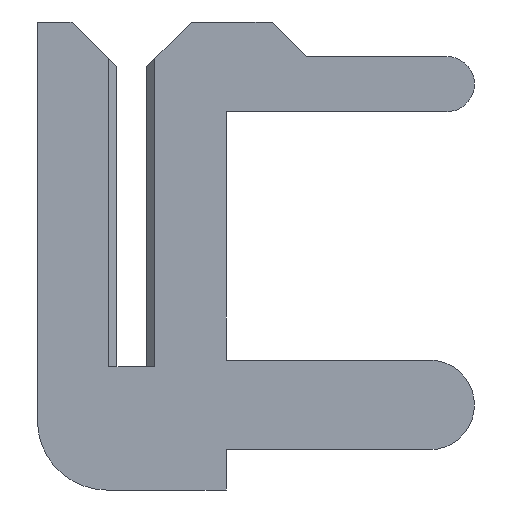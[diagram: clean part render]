
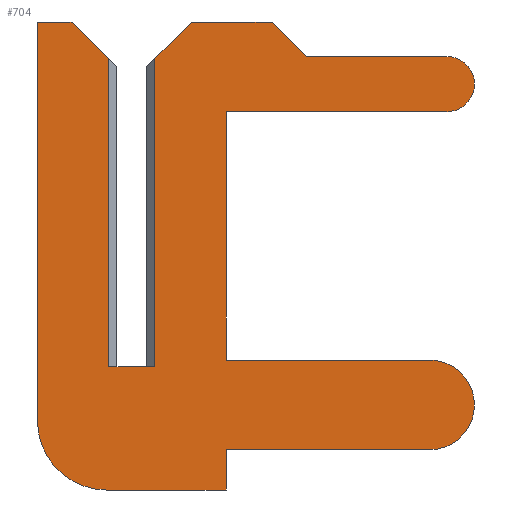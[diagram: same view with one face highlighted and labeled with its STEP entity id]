
A CAD part, left-side view. The second image highlights one B-rep face of the part: STEP entity #704.
In plain terms, the highlighted planar face has unit normal (-1, 0, 0).
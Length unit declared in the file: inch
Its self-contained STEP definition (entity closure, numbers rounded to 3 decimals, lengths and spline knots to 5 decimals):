
#10 = DIRECTION ( 'NONE',  ( 0., -1., 0. ) ) ;
#14 = ORIENTED_EDGE ( 'NONE', *, *, #874, .F. ) ;
#32 = PLANE ( 'NONE',  #618 ) ;
#52 = VERTEX_POINT ( 'NONE', #61 ) ;
#55 = EDGE_CURVE ( 'NONE', #274, #989, #487, .T. ) ;
#57 = VECTOR ( 'NONE', #414, 39.37008 ) ;
#61 = CARTESIAN_POINT ( 'NONE',  ( -0.01, -0.01, 0.134 ) ) ;
#77 = CARTESIAN_POINT ( 'NONE',  ( -0.01, -0.1295, 0.003 ) ) ;
#81 = VERTEX_POINT ( 'NONE', #761 ) ;
#87 = AXIS2_PLACEMENT_3D ( 'NONE', #1028, #701, #204 ) ;
#99 = DIRECTION ( 'NONE',  ( 0., 0., 1. ) ) ;
#117 = LINE ( 'NONE', #719, #149 ) ;
#140 = VECTOR ( 'NONE', #871, 39.37008 ) ;
#149 = VECTOR ( 'NONE', #219, 39.37008 ) ;
#153 = LINE ( 'NONE', #344, #800 ) ;
#162 = VERTEX_POINT ( 'NONE', #771 ) ;
#165 = DIRECTION ( 'NONE',  ( 0., 0., 1. ) ) ;
#181 = ORIENTED_EDGE ( 'NONE', *, *, #519, .F. ) ;
#186 = LINE ( 'NONE', #328, #364 ) ;
#188 = CARTESIAN_POINT ( 'NONE',  ( -0.01, -0.01, 0.15 ) ) ;
#191 = CARTESIAN_POINT ( 'NONE',  ( -0.01, -0.041, -0.0535 ) ) ;
#192 = CARTESIAN_POINT ( 'NONE',  ( -0.01, 0.01, 0. ) ) ;
#195 = VERTEX_POINT ( 'NONE', #383 ) ;
#197 = VERTEX_POINT ( 'NONE', #1095 ) ;
#199 = ORIENTED_EDGE ( 'NONE', *, *, #672, .F. ) ;
#200 = CIRCLE ( 'NONE', #1031, 0.012 ) ;
#204 = DIRECTION ( 'NONE',  ( 0., 0., 1. ) ) ;
#212 = CARTESIAN_POINT ( 'NONE',  ( -0.01, -0.041, -0.0535 ) ) ;
#213 = VECTOR ( 'NONE', #10, 39.37008 ) ;
#219 = DIRECTION ( 'NONE',  ( 0., 1., 0. ) ) ;
#226 = DIRECTION ( 'NONE',  ( 0., 1., 0. ) ) ;
#237 = DIRECTION ( 'NONE',  ( 0., 0., 1. ) ) ;
#272 = DIRECTION ( 'NONE',  ( 0., -0.707, -0.707 ) ) ;
#274 = VERTEX_POINT ( 'NONE', #192 ) ;
#275 = VERTEX_POINT ( 'NONE', #1210 ) ;
#299 = EDGE_CURVE ( 'NONE', #275, #1102, #401, .T. ) ;
#300 = CARTESIAN_POINT ( 'NONE',  ( -0.01, -0.137, 0.111 ) ) ;
#313 = VECTOR ( 'NONE', #165, 39.37008 ) ;
#328 = CARTESIAN_POINT ( 'NONE',  ( -0.01, -0.076, 0.135 ) ) ;
#343 = ORIENTED_EDGE ( 'NONE', *, *, #1260, .F. ) ;
#344 = CARTESIAN_POINT ( 'NONE',  ( -0.01, -0.041, -0.036 ) ) ;
#353 = LINE ( 'NONE', #1224, #926 ) ;
#364 = VECTOR ( 'NONE', #1034, 39.37008 ) ;
#368 = CARTESIAN_POINT ( 'NONE',  ( -0.01, 0.0065, 0.1305 ) ) ;
#369 = VECTOR ( 'NONE', #1001, 39.37008 ) ;
#370 = DIRECTION ( 'NONE',  ( 0., -1., 0. ) ) ;
#371 = ORIENTED_EDGE ( 'NONE', *, *, #504, .T. ) ;
#383 = CARTESIAN_POINT ( 'NONE',  ( -0.01, 0.041, -0.0235 ) ) ;
#384 = ORIENTED_EDGE ( 'NONE', *, *, #547, .F. ) ;
#391 = VECTOR ( 'NONE', #1147, 39.37008 ) ;
#394 = CARTESIAN_POINT ( 'NONE',  ( -0.01, -0.137, 0.123 ) ) ;
#401 = LINE ( 'NONE', #77, #369 ) ;
#414 = DIRECTION ( 'NONE',  ( 0., 0., -1. ) ) ;
#419 = ORIENTED_EDGE ( 'NONE', *, *, #739, .F. ) ;
#421 = DIRECTION ( 'NONE',  ( 0., 0., -1. ) ) ;
#441 = ORIENTED_EDGE ( 'NONE', *, *, #55, .F. ) ;
#444 = CARTESIAN_POINT ( 'NONE',  ( -0.01, 0.011, -0.0235 ) ) ;
#462 = LINE ( 'NONE', #1049, #391 ) ;
#477 = LINE ( 'NONE', #368, #671 ) ;
#487 = LINE ( 'NONE', #961, #140 ) ;
#496 = LINE ( 'NONE', #188, #864 ) ;
#504 = EDGE_CURVE ( 'NONE', #274, #162, #582, .T. ) ;
#518 = VERTEX_POINT ( 'NONE', #1127 ) ;
#519 = EDGE_CURVE ( 'NONE', #1248, #1035, #353, .T. ) ;
#530 = VERTEX_POINT ( 'NONE', #1228 ) ;
#547 = EDGE_CURVE ( 'NONE', #791, #1081, #568, .T. ) ;
#565 = EDGE_LOOP ( 'NONE', ( #1098, #603, #441, #371, #819, #181, #14, #636, #419, #384, #1231, #709, #652, #199, #638, #726, #343, #1037, #821 ) ) ;
#568 = LINE ( 'NONE', #212, #57 ) ;
#570 = CARTESIAN_POINT ( 'NONE',  ( -0.01, -0.1295, -0.036 ) ) ;
#582 = LINE ( 'NONE', #900, #1268 ) ;
#603 = ORIENTED_EDGE ( 'NONE', *, *, #1197, .T. ) ;
#605 = EDGE_CURVE ( 'NONE', #1102, #953, #891, .T. ) ;
#618 = AXIS2_PLACEMENT_3D ( 'NONE', #444, #660, #237 ) ;
#636 = ORIENTED_EDGE ( 'NONE', *, *, #1267, .F. ) ;
#638 = ORIENTED_EDGE ( 'NONE', *, *, #1160, .F. ) ;
#644 = LINE ( 'NONE', #1236, #213 ) ;
#652 = ORIENTED_EDGE ( 'NONE', *, *, #299, .F. ) ;
#660 = DIRECTION ( 'NONE',  ( -1., 0., 0. ) ) ;
#670 = VERTEX_POINT ( 'NONE', #905 ) ;
#671 = VECTOR ( 'NONE', #272, 39.37008 ) ;
#672 = EDGE_CURVE ( 'NONE', #530, #275, #994, .T. ) ;
#675 = VECTOR ( 'NONE', #883, 39.37008 ) ;
#701 = DIRECTION ( 'NONE',  ( 1., 0., 0. ) ) ;
#704 = ADVANCED_FACE ( 'NONE', ( #711 ), #32, .T. ) ;
#706 = EDGE_CURVE ( 'NONE', #52, #518, #462, .T. ) ;
#709 = ORIENTED_EDGE ( 'NONE', *, *, #605, .F. ) ;
#711 = FACE_OUTER_BOUND ( 'NONE', #565, .T. ) ;
#719 = CARTESIAN_POINT ( 'NONE',  ( -0.01, 0.011, -0.0535 ) ) ;
#726 = ORIENTED_EDGE ( 'NONE', *, *, #1062, .F. ) ;
#738 = CARTESIAN_POINT ( 'NONE',  ( -0.01, -0.041, 0.003 ) ) ;
#739 = EDGE_CURVE ( 'NONE', #1081, #744, #117, .T. ) ;
#744 = VERTEX_POINT ( 'NONE', #1040 ) ;
#761 = CARTESIAN_POINT ( 'NONE',  ( -0.01, -0.137, 0.135 ) ) ;
#764 = CARTESIAN_POINT ( 'NONE',  ( -0.01, -0.026, 0.15 ) ) ;
#767 = VECTOR ( 'NONE', #370, 39.37008 ) ;
#771 = CARTESIAN_POINT ( 'NONE',  ( -0.01, 0.01, 0.134 ) ) ;
#785 = CARTESIAN_POINT ( 'NONE',  ( -0.01, -0.041, 0.111 ) ) ;
#791 = VERTEX_POINT ( 'NONE', #940 ) ;
#798 = EDGE_CURVE ( 'NONE', #670, #197, #186, .T. ) ;
#800 = VECTOR ( 'NONE', #226, 39.37008 ) ;
#808 = DIRECTION ( 'NONE',  ( 0., 0., 1. ) ) ;
#819 = ORIENTED_EDGE ( 'NONE', *, *, #968, .F. ) ;
#821 = ORIENTED_EDGE ( 'NONE', *, *, #830, .F. ) ;
#826 = LINE ( 'NONE', #764, #767 ) ;
#830 = EDGE_CURVE ( 'NONE', #518, #670, #826, .T. ) ;
#864 = VECTOR ( 'NONE', #421, 39.37008 ) ;
#866 = CARTESIAN_POINT ( 'NONE',  ( -0.01, 0.041, 0.15 ) ) ;
#871 = DIRECTION ( 'NONE',  ( 0., -1., 0. ) ) ;
#874 = EDGE_CURVE ( 'NONE', #195, #1248, #1285, .T. ) ;
#883 = DIRECTION ( 'NONE',  ( 0., 1., 0. ) ) ;
#891 = CIRCLE ( 'NONE', #1150, 0.0195 ) ;
#898 = CARTESIAN_POINT ( 'NONE',  ( -0.01, -0.1295, 0.003 ) ) ;
#900 = CARTESIAN_POINT ( 'NONE',  ( -0.01, 0.01, -0.0235 ) ) ;
#905 = CARTESIAN_POINT ( 'NONE',  ( -0.01, -0.061, 0.15 ) ) ;
#910 = CARTESIAN_POINT ( 'NONE',  ( -0.01, 0.041, 0.15 ) ) ;
#926 = VECTOR ( 'NONE', #1220, 39.37008 ) ;
#940 = CARTESIAN_POINT ( 'NONE',  ( -0.01, -0.041, -0.036 ) ) ;
#953 = VERTEX_POINT ( 'NONE', #570 ) ;
#961 = CARTESIAN_POINT ( 'NONE',  ( -0.01, 0.0065, 0. ) ) ;
#968 = EDGE_CURVE ( 'NONE', #1035, #162, #477, .T. ) ;
#989 = VERTEX_POINT ( 'NONE', #1008 ) ;
#994 = LINE ( 'NONE', #738, #1011 ) ;
#1001 = DIRECTION ( 'NONE',  ( 0., -1., 0. ) ) ;
#1003 = DIRECTION ( 'NONE',  ( 0., 0., 1. ) ) ;
#1008 = CARTESIAN_POINT ( 'NONE',  ( -0.01, -0.01, 0. ) ) ;
#1011 = VECTOR ( 'NONE', #1237, 39.37008 ) ;
#1024 = CARTESIAN_POINT ( 'NONE',  ( -0.01, -0.1295, -0.0165 ) ) ;
#1028 = CARTESIAN_POINT ( 'NONE',  ( -0.01, 0.011, -0.0235 ) ) ;
#1031 = AXIS2_PLACEMENT_3D ( 'NONE', #394, #1100, #1003 ) ;
#1034 = DIRECTION ( 'NONE',  ( 0., -0.707, -0.707 ) ) ;
#1035 = VERTEX_POINT ( 'NONE', #1090 ) ;
#1037 = ORIENTED_EDGE ( 'NONE', *, *, #798, .F. ) ;
#1040 = CARTESIAN_POINT ( 'NONE',  ( -0.01, 0.011, -0.0535 ) ) ;
#1049 = CARTESIAN_POINT ( 'NONE',  ( -0.01, -0.0065, 0.1305 ) ) ;
#1062 = EDGE_CURVE ( 'NONE', #81, #1245, #200, .T. ) ;
#1081 = VERTEX_POINT ( 'NONE', #191 ) ;
#1090 = CARTESIAN_POINT ( 'NONE',  ( -0.01, 0.026, 0.15 ) ) ;
#1095 = CARTESIAN_POINT ( 'NONE',  ( -0.01, -0.076, 0.135 ) ) ;
#1098 = ORIENTED_EDGE ( 'NONE', *, *, #706, .F. ) ;
#1100 = DIRECTION ( 'NONE',  ( 1., 0., 0. ) ) ;
#1102 = VERTEX_POINT ( 'NONE', #898 ) ;
#1112 = DIRECTION ( 'NONE',  ( 1., 0., 0. ) ) ;
#1127 = CARTESIAN_POINT ( 'NONE',  ( -0.01, -0.026, 0.15 ) ) ;
#1144 = LINE ( 'NONE', #785, #675 ) ;
#1147 = DIRECTION ( 'NONE',  ( 0., -0.707, 0.707 ) ) ;
#1150 = AXIS2_PLACEMENT_3D ( 'NONE', #1024, #1112, #99 ) ;
#1160 = EDGE_CURVE ( 'NONE', #1245, #530, #1144, .T. ) ;
#1163 = CIRCLE ( 'NONE', #87, 0.03 ) ;
#1197 = EDGE_CURVE ( 'NONE', #52, #989, #496, .T. ) ;
#1210 = CARTESIAN_POINT ( 'NONE',  ( -0.01, -0.041, 0.003 ) ) ;
#1220 = DIRECTION ( 'NONE',  ( 0., -1., 0. ) ) ;
#1224 = CARTESIAN_POINT ( 'NONE',  ( -0.01, 0.026, 0.15 ) ) ;
#1228 = CARTESIAN_POINT ( 'NONE',  ( -0.01, -0.041, 0.111 ) ) ;
#1231 = ORIENTED_EDGE ( 'NONE', *, *, #1314, .F. ) ;
#1236 = CARTESIAN_POINT ( 'NONE',  ( -0.01, -0.137, 0.135 ) ) ;
#1237 = DIRECTION ( 'NONE',  ( 0., 0., -1. ) ) ;
#1245 = VERTEX_POINT ( 'NONE', #300 ) ;
#1248 = VERTEX_POINT ( 'NONE', #910 ) ;
#1260 = EDGE_CURVE ( 'NONE', #197, #81, #644, .T. ) ;
#1267 = EDGE_CURVE ( 'NONE', #744, #195, #1163, .T. ) ;
#1268 = VECTOR ( 'NONE', #808, 39.37008 ) ;
#1285 = LINE ( 'NONE', #866, #313 ) ;
#1314 = EDGE_CURVE ( 'NONE', #953, #791, #153, .T. ) ;
